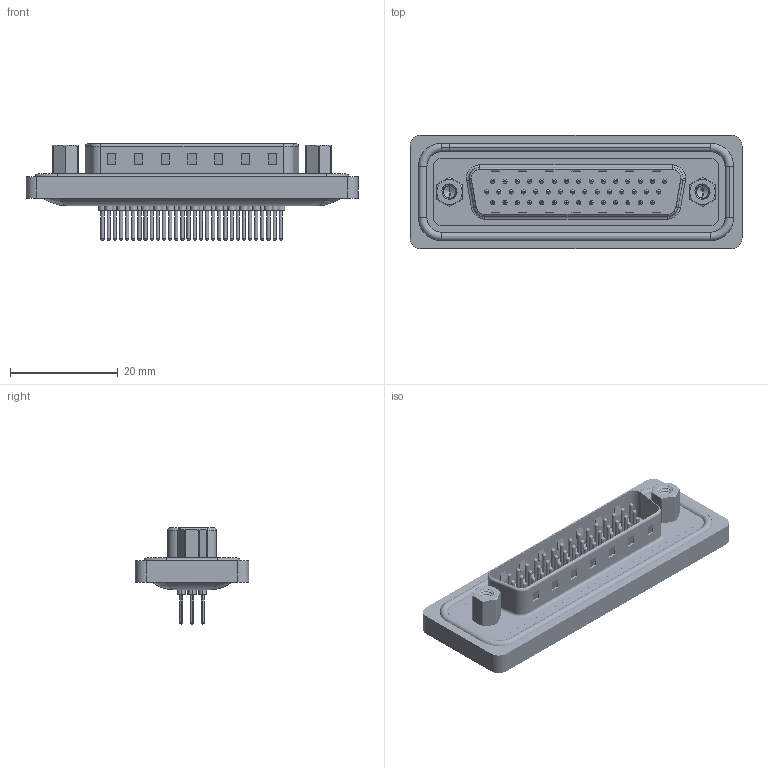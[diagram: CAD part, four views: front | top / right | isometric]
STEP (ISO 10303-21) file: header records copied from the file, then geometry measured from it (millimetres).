
FILE_DESCRIPTION (( 'STEP AP203' ), '1' );
FILE_NAME ('637-W44-221-012.STEP', '2018-11-28T16:34:09', ( '' ), ( '' ), 'SwSTEP 2.0', 'SolidWorks 2016', '' );
FILE_SCHEMA (( 'CONFIG_CONTROL_DESIGN' ));
Length unit declared in the file: millimetre
Products named in the file (9): 637-W44-221-012; 637W Housing_44 Contacts; 637W Shell_44 Contacts; 637W Contact Row 1_21; 637W Contact Row 2_21; 637W Contact Row 3_21; 637W Waterproof Housing_44 Contacts; 637W 4-40 Threaded Rivet; 637W 4-40 Hex Standoff
Assembly tree (51 placements, depth 2):
  637-W44-221-012
    637W Housing_44 Contacts
    637W Shell_44 Contacts
    637W Contact Row 1_21  x15
    637W Contact Row 2_21  x15
    637W Contact Row 3_21  x14
    637W Waterproof Housing_44 Contacts
    637W 4-40 Threaded Rivet  x2
    637W 4-40 Hex Standoff  x2
Bounding box: 61.74 x 21.1 x 17.9 mm (x, y, z)
Volume: 6371.9 mm3; surface area: 12028.3 mm2
Topology: 52 solids, 52 shells, 2234 faces, 4870 edges, 2971 vertices
Faces by surface type: cylinder 920, torus 747, plane 513, cone 32, bspline 22
Entity records: 35182 total; most frequent: CARTESIAN_POINT 9433, DIRECTION 5320, ORIENTED_EDGE 4626, EDGE_CURVE 2313, AXIS2_PLACEMENT_3D 2160, VERTEX_POINT 1494, EDGE_LOOP 1275, CIRCLE 1170
